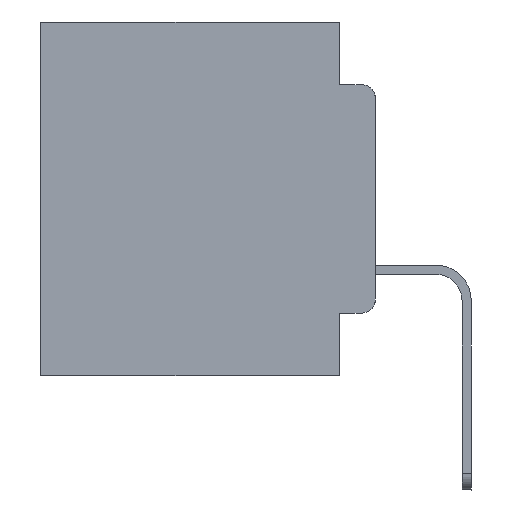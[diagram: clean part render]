
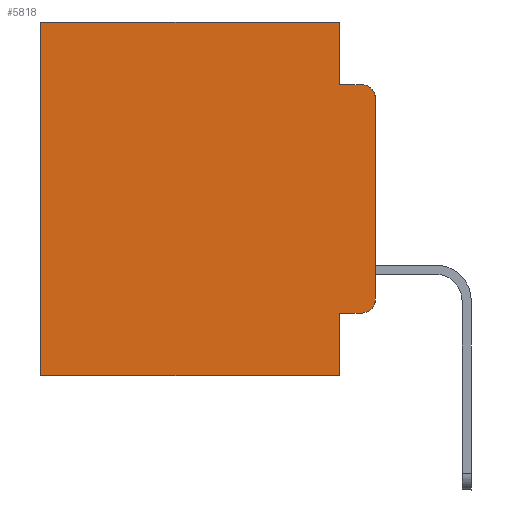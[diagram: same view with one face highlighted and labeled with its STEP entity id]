
A CAD part, left-side view. The second image highlights one B-rep face of the part: STEP entity #5818.
In plain terms, the highlighted planar face has unit normal (-1, 0, 0).
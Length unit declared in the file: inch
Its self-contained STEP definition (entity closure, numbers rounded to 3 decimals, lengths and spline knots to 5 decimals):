
#499 = ORIENTED_EDGE ( 'NONE', *, *, #13084, .F. ) ;
#513 = LINE ( 'NONE', #22197, #17258 ) ;
#643 = CARTESIAN_POINT ( 'NONE',  ( 0.298, 0.051, 0. ) ) ;
#901 = ORIENTED_EDGE ( 'NONE', *, *, #8475, .F. ) ;
#1521 = ORIENTED_EDGE ( 'NONE', *, *, #12644, .F. ) ;
#1686 = CARTESIAN_POINT ( 'NONE',  ( 0.298, 0.473, 0. ) ) ;
#1906 = LINE ( 'NONE', #8689, #24000 ) ;
#2008 = LINE ( 'NONE', #6734, #15720 ) ;
#2197 = EDGE_LOOP ( 'NONE', ( #901, #9549, #1521, #22947, #19941, #16795, #23645, #499, #9236, #17730 ) ) ;
#2235 = DIRECTION ( 'NONE',  ( 0., 1., 0. ) ) ;
#2367 = VERTEX_POINT ( 'NONE', #3177 ) ;
#2526 = PLANE ( 'NONE',  #24969 ) ;
#3149 = VERTEX_POINT ( 'NONE', #643 ) ;
#3177 = CARTESIAN_POINT ( 'NONE',  ( 0.298, 0.051, -0.4115 ) ) ;
#3514 = CARTESIAN_POINT ( 'NONE',  ( 0.298, 0.473, 0. ) ) ;
#4075 = EDGE_CURVE ( 'NONE', #26194, #4216, #5267, .T. ) ;
#4216 = VERTEX_POINT ( 'NONE', #26631 ) ;
#4259 = VERTEX_POINT ( 'NONE', #13898 ) ;
#4655 = EDGE_CURVE ( 'NONE', #3149, #18541, #1906, .T. ) ;
#4783 = CARTESIAN_POINT ( 'NONE',  ( 0.298, 0., -0.1085 ) ) ;
#5267 = CIRCLE ( 'NONE', #26720, 0.02 ) ;
#5532 = CARTESIAN_POINT ( 'NONE',  ( 0.298, 0.473, -0.5 ) ) ;
#5818 = ADVANCED_FACE ( 'NONE', ( #23309 ), #2526, .F. ) ;
#6065 = DIRECTION ( 'NONE',  ( 0., -1., 0. ) ) ;
#6734 = CARTESIAN_POINT ( 'NONE',  ( 0.298, 0., -0.5 ) ) ;
#6911 = DIRECTION ( 'NONE',  ( 0., 0., -1. ) ) ;
#7256 = LINE ( 'NONE', #18339, #18657 ) ;
#7701 = CARTESIAN_POINT ( 'NONE',  ( 0.298, 0.02, -0.1085 ) ) ;
#7746 = DIRECTION ( 'NONE',  ( 0., 0., -1. ) ) ;
#8475 = EDGE_CURVE ( 'NONE', #26194, #25605, #10115, .T. ) ;
#8689 = CARTESIAN_POINT ( 'NONE',  ( 0.298, 0., 0. ) ) ;
#9236 = ORIENTED_EDGE ( 'NONE', *, *, #13985, .T. ) ;
#9549 = ORIENTED_EDGE ( 'NONE', *, *, #4075, .T. ) ;
#10115 = LINE ( 'NONE', #18605, #14133 ) ;
#10919 = LINE ( 'NONE', #24483, #21635 ) ;
#11985 = EDGE_CURVE ( 'NONE', #3149, #14682, #7256, .T. ) ;
#12531 = VERTEX_POINT ( 'NONE', #15872 ) ;
#12644 = EDGE_CURVE ( 'NONE', #14682, #4216, #10919, .T. ) ;
#13084 = EDGE_CURVE ( 'NONE', #2367, #4259, #513, .T. ) ;
#13240 = VERTEX_POINT ( 'NONE', #5532 ) ;
#13264 = DIRECTION ( 'NONE',  ( 0., 1., 0. ) ) ;
#13440 = CIRCLE ( 'NONE', #15865, 0.02 ) ;
#13492 = CARTESIAN_POINT ( 'NONE',  ( 0.298, 0.02, -0.3915 ) ) ;
#13898 = CARTESIAN_POINT ( 'NONE',  ( 0.298, 0.051, -0.5 ) ) ;
#13985 = EDGE_CURVE ( 'NONE', #2367, #12531, #25416, .T. ) ;
#14133 = VECTOR ( 'NONE', #7746, 39.37008 ) ;
#14682 = VERTEX_POINT ( 'NONE', #27734 ) ;
#15720 = VECTOR ( 'NONE', #13264, 39.37008 ) ;
#15865 = AXIS2_PLACEMENT_3D ( 'NONE', #13492, #20154, #22117 ) ;
#15872 = CARTESIAN_POINT ( 'NONE',  ( 0.298, 0.02, -0.4115 ) ) ;
#16038 = VECTOR ( 'NONE', #6065, 39.37008 ) ;
#16795 = ORIENTED_EDGE ( 'NONE', *, *, #22870, .T. ) ;
#17258 = VECTOR ( 'NONE', #17920, 39.37008 ) ;
#17377 = LINE ( 'NONE', #3514, #22372 ) ;
#17730 = ORIENTED_EDGE ( 'NONE', *, *, #25673, .T. ) ;
#17920 = DIRECTION ( 'NONE',  ( 0., 0., -1. ) ) ;
#18339 = CARTESIAN_POINT ( 'NONE',  ( 0.298, 0.051, 0. ) ) ;
#18541 = VERTEX_POINT ( 'NONE', #1686 ) ;
#18605 = CARTESIAN_POINT ( 'NONE',  ( 0.298, 0., 0. ) ) ;
#18657 = VECTOR ( 'NONE', #20478, 39.37008 ) ;
#18983 = CARTESIAN_POINT ( 'NONE',  ( 0.298, 0.051, -0.4115 ) ) ;
#19434 = CARTESIAN_POINT ( 'NONE',  ( 0.298, 0., -0.3915 ) ) ;
#19941 = ORIENTED_EDGE ( 'NONE', *, *, #4655, .T. ) ;
#20154 = DIRECTION ( 'NONE',  ( -1., 0., 0. ) ) ;
#20478 = DIRECTION ( 'NONE',  ( 0., 0., -1. ) ) ;
#20993 = DIRECTION ( 'NONE',  ( 0., 0., -1. ) ) ;
#21513 = CARTESIAN_POINT ( 'NONE',  ( 0.298, 0., 0. ) ) ;
#21635 = VECTOR ( 'NONE', #24196, 39.37008 ) ;
#21968 = EDGE_CURVE ( 'NONE', #4259, #13240, #2008, .T. ) ;
#22117 = DIRECTION ( 'NONE',  ( 0., 0., -1. ) ) ;
#22197 = CARTESIAN_POINT ( 'NONE',  ( 0.298, 0.051, 0. ) ) ;
#22372 = VECTOR ( 'NONE', #20993, 39.37008 ) ;
#22674 = DIRECTION ( 'NONE',  ( -1., 0., 0. ) ) ;
#22870 = EDGE_CURVE ( 'NONE', #18541, #13240, #17377, .T. ) ;
#22947 = ORIENTED_EDGE ( 'NONE', *, *, #11985, .F. ) ;
#23309 = FACE_OUTER_BOUND ( 'NONE', #2197, .T. ) ;
#23645 = ORIENTED_EDGE ( 'NONE', *, *, #21968, .F. ) ;
#24000 = VECTOR ( 'NONE', #2235, 39.37008 ) ;
#24196 = DIRECTION ( 'NONE',  ( 0., -1., 0. ) ) ;
#24483 = CARTESIAN_POINT ( 'NONE',  ( 0.298, 0.051, -0.0885 ) ) ;
#24969 = AXIS2_PLACEMENT_3D ( 'NONE', #21513, #26091, #6911 ) ;
#25009 = DIRECTION ( 'NONE',  ( 0., 0., -1. ) ) ;
#25416 = LINE ( 'NONE', #18983, #16038 ) ;
#25605 = VERTEX_POINT ( 'NONE', #19434 ) ;
#25673 = EDGE_CURVE ( 'NONE', #12531, #25605, #13440, .T. ) ;
#26091 = DIRECTION ( 'NONE',  ( 1., 0., 0. ) ) ;
#26194 = VERTEX_POINT ( 'NONE', #4783 ) ;
#26631 = CARTESIAN_POINT ( 'NONE',  ( 0.298, 0.02, -0.0885 ) ) ;
#26720 = AXIS2_PLACEMENT_3D ( 'NONE', #7701, #22674, #25009 ) ;
#27734 = CARTESIAN_POINT ( 'NONE',  ( 0.298, 0.051, -0.0885 ) ) ;
